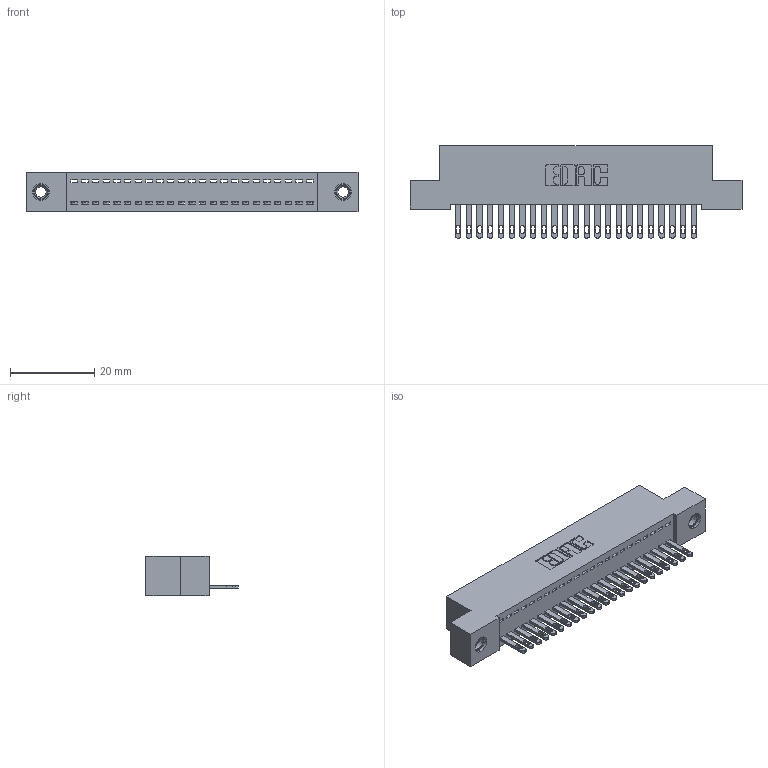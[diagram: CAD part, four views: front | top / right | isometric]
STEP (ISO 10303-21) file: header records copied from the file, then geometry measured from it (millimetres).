
FILE_DESCRIPTION (( 'STEP AP203' ), '1' );
FILE_NAME ('342-023-500-107.STEP', '2019-10-01T22:59:13', ( '' ), ( '' ), 'SwSTEP 2.0', 'SolidWorks 2016', '' );
FILE_SCHEMA (( 'CONFIG_CONTROL_DESIGN' ));
Length unit declared in the file: inch
Products named in the file (4): 345-292-001_345-293-100; 345-250-001_345-250-005-103; 342-023-500-107; 342 Part_TI
Assembly tree (26 placements, depth 2):
  342-023-500-107
    342 Part_TI
    345-292-001_345-293-100  x23
    345-250-001_345-250-005-103  x2
Bounding box: 78.74 x 21.85 x 9.4 mm (x, y, z)
Volume: 6835.5 mm3; surface area: 9760.3 mm2
Topology: 26 solids, 26 shells, 1412 faces, 4299 edges, 2858 vertices
Faces by surface type: plane 926, cylinder 470, cone 12, torus 4
Entity records: 17502 total; most frequent: CARTESIAN_POINT 3002, ORIENTED_EDGE 2954, DIRECTION 2605, EDGE_CURVE 1477, VECTOR 1325, LINE 1325, VERTEX_POINT 980, AXIS2_PLACEMENT_3D 640
